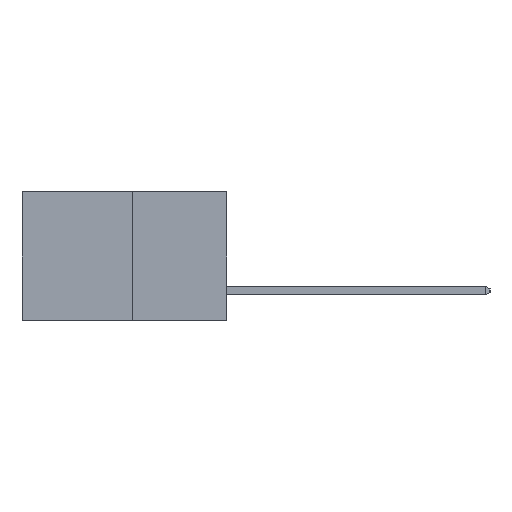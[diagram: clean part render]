
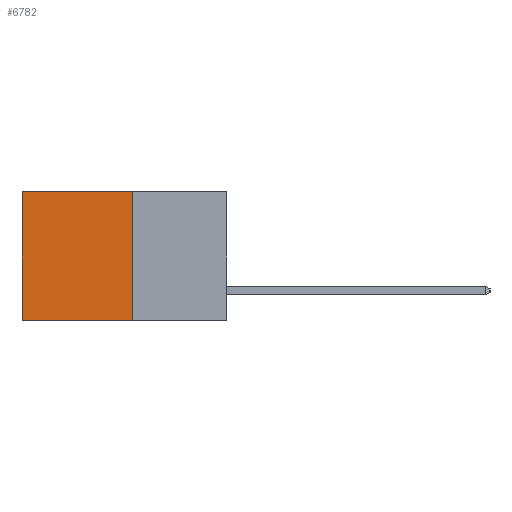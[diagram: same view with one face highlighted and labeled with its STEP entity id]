
A CAD part, left-side view. The second image highlights one B-rep face of the part: STEP entity #6782.
In plain terms, the highlighted planar face has unit normal (-1, 0, 0).
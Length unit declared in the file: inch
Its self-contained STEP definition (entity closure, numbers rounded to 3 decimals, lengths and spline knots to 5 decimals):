
#289 = VECTOR ( 'NONE', #1219, 39.37008 ) ;
#293 = CARTESIAN_POINT ( 'NONE',  ( 0.277, 0.27, -0.37 ) ) ;
#576 = CARTESIAN_POINT ( 'NONE',  ( 0.277, 0.27, -0.37 ) ) ;
#1031 = CARTESIAN_POINT ( 'NONE',  ( 0.277, 0.27, -0.37 ) ) ;
#1173 = ORIENTED_EDGE ( 'NONE', *, *, #10311, .F. ) ;
#1193 = LINE ( 'NONE', #6921, #5583 ) ;
#1219 = DIRECTION ( 'NONE',  ( 0., 0., -1. ) ) ;
#1449 = CARTESIAN_POINT ( 'NONE',  ( 0.277, 0.59, -0.37 ) ) ;
#1888 = VERTEX_POINT ( 'NONE', #4374 ) ;
#2112 = DIRECTION ( 'NONE',  ( 0., 1., 0. ) ) ;
#2434 = ORIENTED_EDGE ( 'NONE', *, *, #9257, .T. ) ;
#2854 = PLANE ( 'NONE',  #3647 ) ;
#3054 = VECTOR ( 'NONE', #8647, 39.37008 ) ;
#3647 = AXIS2_PLACEMENT_3D ( 'NONE', #293, #8389, #3701 ) ;
#3701 = DIRECTION ( 'NONE',  ( 0., 0., -1. ) ) ;
#4228 = EDGE_CURVE ( 'NONE', #8732, #1888, #4744, .T. ) ;
#4374 = CARTESIAN_POINT ( 'NONE',  ( 0.277, 0.59, -0.37 ) ) ;
#4708 = ORIENTED_EDGE ( 'NONE', *, *, #5041, .F. ) ;
#4744 = LINE ( 'NONE', #1449, #289 ) ;
#4772 = VERTEX_POINT ( 'NONE', #9280 ) ;
#5041 = EDGE_CURVE ( 'NONE', #8501, #1888, #5700, .T. ) ;
#5461 = CARTESIAN_POINT ( 'NONE',  ( 0.277, 0.59, 0. ) ) ;
#5583 = VECTOR ( 'NONE', #2112, 39.37008 ) ;
#5700 = LINE ( 'NONE', #8677, #3054 ) ;
#6301 = DIRECTION ( 'NONE',  ( 0., 0., -1. ) ) ;
#6782 = ADVANCED_FACE ( 'NONE', ( #7258 ), #2854, .F. ) ;
#6801 = ORIENTED_EDGE ( 'NONE', *, *, #4228, .T. ) ;
#6921 = CARTESIAN_POINT ( 'NONE',  ( 0.277, 0.27, 0. ) ) ;
#7258 = FACE_OUTER_BOUND ( 'NONE', #9959, .T. ) ;
#8389 = DIRECTION ( 'NONE',  ( 1., 0., 0. ) ) ;
#8501 = VERTEX_POINT ( 'NONE', #1031 ) ;
#8647 = DIRECTION ( 'NONE',  ( 0., 1., 0. ) ) ;
#8677 = CARTESIAN_POINT ( 'NONE',  ( 0.277, 0.27, -0.37 ) ) ;
#8732 = VERTEX_POINT ( 'NONE', #5461 ) ;
#8845 = LINE ( 'NONE', #576, #9795 ) ;
#9257 = EDGE_CURVE ( 'NONE', #4772, #8732, #1193, .T. ) ;
#9280 = CARTESIAN_POINT ( 'NONE',  ( 0.277, 0.27, 0. ) ) ;
#9795 = VECTOR ( 'NONE', #6301, 39.37008 ) ;
#9959 = EDGE_LOOP ( 'NONE', ( #6801, #4708, #1173, #2434 ) ) ;
#10311 = EDGE_CURVE ( 'NONE', #4772, #8501, #8845, .T. ) ;
